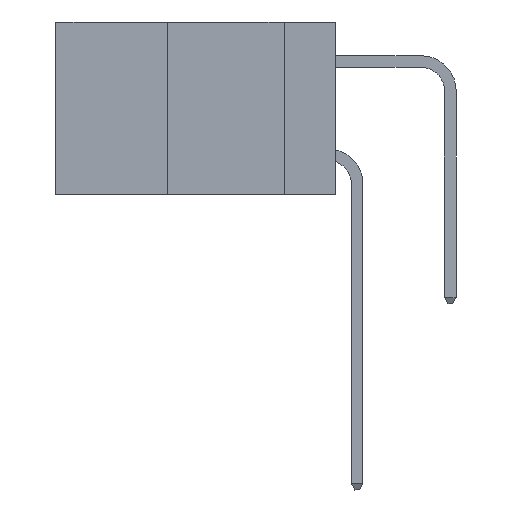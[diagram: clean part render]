
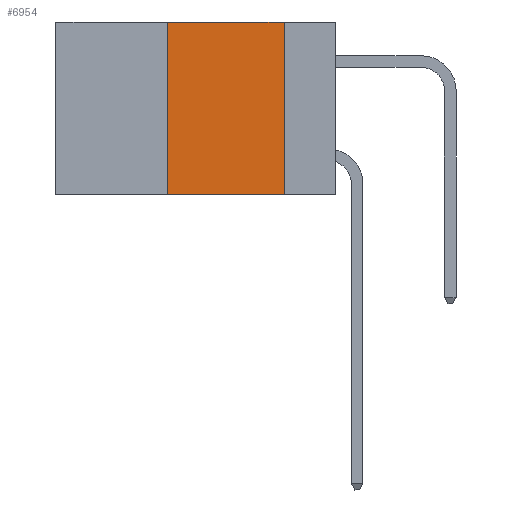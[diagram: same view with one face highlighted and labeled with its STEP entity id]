
A CAD part, left-side view. The second image highlights one B-rep face of the part: STEP entity #6954.
In plain terms, the highlighted planar face has unit normal (-1, 0, 0).
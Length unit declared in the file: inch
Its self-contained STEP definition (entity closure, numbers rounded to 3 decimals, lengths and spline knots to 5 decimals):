
#501 = DIRECTION ( 'NONE',  ( 0., 0., -1. ) ) ;
#943 = CARTESIAN_POINT ( 'NONE',  ( 0., 0.11, 0. ) ) ;
#1232 = VERTEX_POINT ( 'NONE', #13100 ) ;
#1686 = VERTEX_POINT ( 'NONE', #21882 ) ;
#1807 = DIRECTION ( 'NONE',  ( 0., 0., 1. ) ) ;
#2299 = ORIENTED_EDGE ( 'NONE', *, *, #17440, .F. ) ;
#2367 = CARTESIAN_POINT ( 'NONE',  ( 0., 0.11, 0. ) ) ;
#2387 = EDGE_CURVE ( 'NONE', #1686, #12714, #22886, .T. ) ;
#3710 = VECTOR ( 'NONE', #4155, 39.37008 ) ;
#4135 = PLANE ( 'NONE',  #4330 ) ;
#4155 = DIRECTION ( 'NONE',  ( 0., -1., 0. ) ) ;
#4330 = AXIS2_PLACEMENT_3D ( 'NONE', #16917, #5972, #18725 ) ;
#5395 = ORIENTED_EDGE ( 'NONE', *, *, #2387, .F. ) ;
#5972 = DIRECTION ( 'NONE',  ( 1., 0., 0. ) ) ;
#6328 = LINE ( 'NONE', #2367, #15506 ) ;
#6954 = ADVANCED_FACE ( 'NONE', ( #21883 ), #4135, .F. ) ;
#7379 = VECTOR ( 'NONE', #1807, 39.37008 ) ;
#11266 = CARTESIAN_POINT ( 'NONE',  ( 0., 0.11, -0.37 ) ) ;
#11533 = CARTESIAN_POINT ( 'NONE',  ( 0., 0.6, -0.37 ) ) ;
#11924 = VERTEX_POINT ( 'NONE', #11266 ) ;
#12351 = LINE ( 'NONE', #12788, #7379 ) ;
#12714 = VERTEX_POINT ( 'NONE', #943 ) ;
#12788 = CARTESIAN_POINT ( 'NONE',  ( 0., 0.36, 0. ) ) ;
#13100 = CARTESIAN_POINT ( 'NONE',  ( 0., 0.36, -0.37 ) ) ;
#13210 = DIRECTION ( 'NONE',  ( 0., -1., 0. ) ) ;
#13742 = CARTESIAN_POINT ( 'NONE',  ( 0., 0.6, 0. ) ) ;
#15227 = ORIENTED_EDGE ( 'NONE', *, *, #16967, .T. ) ;
#15506 = VECTOR ( 'NONE', #501, 39.37008 ) ;
#15784 = EDGE_CURVE ( 'NONE', #12714, #11924, #6328, .T. ) ;
#16917 = CARTESIAN_POINT ( 'NONE',  ( 0., 0.6, 0. ) ) ;
#16967 = EDGE_CURVE ( 'NONE', #1232, #11924, #23586, .T. ) ;
#17440 = EDGE_CURVE ( 'NONE', #1232, #1686, #12351, .T. ) ;
#18159 = VECTOR ( 'NONE', #13210, 39.37008 ) ;
#18582 = ORIENTED_EDGE ( 'NONE', *, *, #15784, .F. ) ;
#18725 = DIRECTION ( 'NONE',  ( 0., 0., -1. ) ) ;
#20337 = EDGE_LOOP ( 'NONE', ( #18582, #5395, #2299, #15227 ) ) ;
#21882 = CARTESIAN_POINT ( 'NONE',  ( 0., 0.36, 0. ) ) ;
#21883 = FACE_OUTER_BOUND ( 'NONE', #20337, .T. ) ;
#22886 = LINE ( 'NONE', #13742, #18159 ) ;
#23586 = LINE ( 'NONE', #11533, #3710 ) ;
